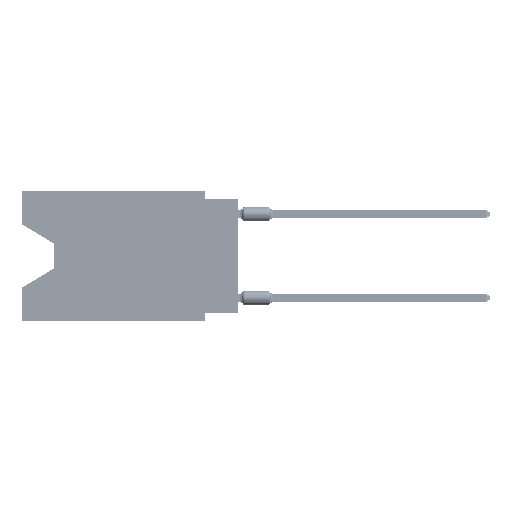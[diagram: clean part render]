
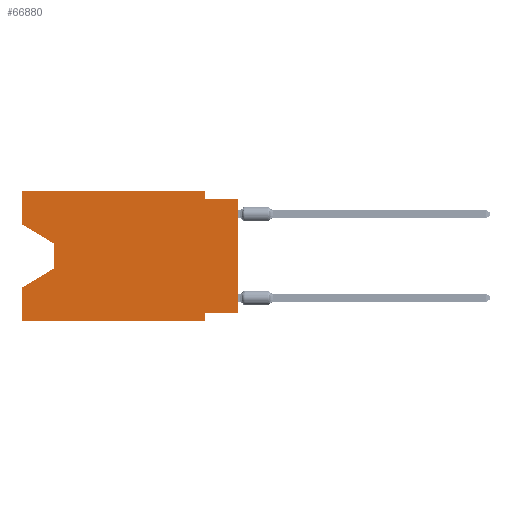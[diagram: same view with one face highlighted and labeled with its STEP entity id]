
A CAD part, left-side view. The second image highlights one B-rep face of the part: STEP entity #66880.
In plain terms, the highlighted planar face has unit normal (-1, 0, 0).
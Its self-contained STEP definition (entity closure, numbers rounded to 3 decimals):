
#413 = EDGE_CURVE ( 'NONE', #23273, #5373, #863, .T. ) ;
#863 = LINE ( 'NONE', #63190, #64928 ) ;
#1180 = DIRECTION ( 'NONE',  ( 0., 0., 1. ) ) ;
#1882 = VERTEX_POINT ( 'NONE', #2113 ) ;
#2113 = CARTESIAN_POINT ( 'NONE',  ( 0., 13.97, -5.893 ) ) ;
#4065 = EDGE_LOOP ( 'NONE', ( #66967, #74789, #69816, #65410, #41796, #32406, #82726, #46219, #72583, #57660, #9290, #78977 ) ) ;
#4071 = VECTOR ( 'NONE', #33538, 1000. ) ;
#5210 = CARTESIAN_POINT ( 'NONE',  ( 0., 16.383, -2.546 ) ) ;
#5373 = VERTEX_POINT ( 'NONE', #28654 ) ;
#8535 = VECTOR ( 'NONE', #65566, 1000. ) ;
#8777 = EDGE_CURVE ( 'NONE', #64967, #54040, #34006, .T. ) ;
#9290 = ORIENTED_EDGE ( 'NONE', *, *, #413, .F. ) ;
#9312 = VERTEX_POINT ( 'NONE', #78275 ) ;
#9584 = LINE ( 'NONE', #36928, #61810 ) ;
#10253 = VECTOR ( 'NONE', #72726, 1000. ) ;
#10540 = DIRECTION ( 'NONE',  ( 0., 0., -1. ) ) ;
#10916 = EDGE_CURVE ( 'NONE', #32950, #16256, #59727, .T. ) ;
#12124 = EDGE_CURVE ( 'NONE', #67497, #31859, #63957, .T. ) ;
#13237 = LINE ( 'NONE', #32962, #67112 ) ;
#13639 = CARTESIAN_POINT ( 'NONE',  ( 0., 0., -0.635 ) ) ;
#16256 = VERTEX_POINT ( 'NONE', #13639 ) ;
#18769 = DIRECTION ( 'NONE',  ( 0., 0., 1. ) ) ;
#19662 = DIRECTION ( 'NONE',  ( 0., -0.855, -0.519 ) ) ;
#20065 = CARTESIAN_POINT ( 'NONE',  ( 0., 16.383, 0. ) ) ;
#20564 = CARTESIAN_POINT ( 'NONE',  ( 0., 16.383, -2.546 ) ) ;
#22253 = CARTESIAN_POINT ( 'NONE',  ( 0., 2.54, -9.906 ) ) ;
#23273 = VERTEX_POINT ( 'NONE', #78458 ) ;
#23763 = FACE_OUTER_BOUND ( 'NONE', #4065, .T. ) ;
#28199 = DIRECTION ( 'NONE',  ( 0., -1., 0. ) ) ;
#28654 = CARTESIAN_POINT ( 'NONE',  ( 0., 2.54, 0. ) ) ;
#28971 = DIRECTION ( 'NONE',  ( 0., 0., -1. ) ) ;
#30026 = VECTOR ( 'NONE', #19662, 1000. ) ;
#31859 = VERTEX_POINT ( 'NONE', #34199 ) ;
#32406 = ORIENTED_EDGE ( 'NONE', *, *, #12124, .F. ) ;
#32950 = VERTEX_POINT ( 'NONE', #40521 ) ;
#32962 = CARTESIAN_POINT ( 'NONE',  ( 0., 16.383, -9.906 ) ) ;
#33538 = DIRECTION ( 'NONE',  ( 0., 0., 1. ) ) ;
#34006 = LINE ( 'NONE', #20564, #30026 ) ;
#34199 = CARTESIAN_POINT ( 'NONE',  ( 0., 2.54, -9.906 ) ) ;
#36928 = CARTESIAN_POINT ( 'NONE',  ( 0., 2.54, 0. ) ) ;
#37374 = DIRECTION ( 'NONE',  ( 0., 0., -1. ) ) ;
#38967 = CARTESIAN_POINT ( 'NONE',  ( 0., 0., -9.271 ) ) ;
#39157 = VERTEX_POINT ( 'NONE', #80428 ) ;
#40521 = CARTESIAN_POINT ( 'NONE',  ( 0., 2.54, -0.635 ) ) ;
#40680 = CARTESIAN_POINT ( 'NONE',  ( 0., 0., 0. ) ) ;
#41796 = ORIENTED_EDGE ( 'NONE', *, *, #63241, .T. ) ;
#43984 = EDGE_CURVE ( 'NONE', #39157, #67497, #69951, .T. ) ;
#44090 = EDGE_CURVE ( 'NONE', #45992, #9312, #46581, .T. ) ;
#44504 = LINE ( 'NONE', #71853, #8535 ) ;
#44846 = DIRECTION ( 'NONE',  ( 0., 0., -1. ) ) ;
#45992 = VERTEX_POINT ( 'NONE', #80542 ) ;
#46219 = ORIENTED_EDGE ( 'NONE', *, *, #68720, .T. ) ;
#46581 = LINE ( 'NONE', #52417, #74179 ) ;
#48721 = EDGE_CURVE ( 'NONE', #54040, #1882, #57646, .T. ) ;
#51124 = PLANE ( 'NONE',  #70439 ) ;
#52417 = CARTESIAN_POINT ( 'NONE',  ( 0., 16.383, 0. ) ) ;
#54040 = VERTEX_POINT ( 'NONE', #62503 ) ;
#57646 = LINE ( 'NONE', #85004, #78488 ) ;
#57660 = ORIENTED_EDGE ( 'NONE', *, *, #73236, .F. ) ;
#59727 = LINE ( 'NONE', #73168, #10253 ) ;
#59914 = VECTOR ( 'NONE', #60021, 1000. ) ;
#60021 = DIRECTION ( 'NONE',  ( 0., 1., 0. ) ) ;
#61230 = EDGE_CURVE ( 'NONE', #64967, #23273, #86924, .T. ) ;
#61810 = VECTOR ( 'NONE', #37374, 1000. ) ;
#62503 = CARTESIAN_POINT ( 'NONE',  ( 0., 13.97, -4.013 ) ) ;
#63190 = CARTESIAN_POINT ( 'NONE',  ( 0., 16.383, 0. ) ) ;
#63241 = EDGE_CURVE ( 'NONE', #45992, #31859, #13237, .T. ) ;
#63396 = CARTESIAN_POINT ( 'NONE',  ( 0., 2.54, -9.271 ) ) ;
#63957 = LINE ( 'NONE', #22253, #78878 ) ;
#64928 = VECTOR ( 'NONE', #28199, 1000. ) ;
#64967 = VERTEX_POINT ( 'NONE', #5210 ) ;
#65410 = ORIENTED_EDGE ( 'NONE', *, *, #44090, .F. ) ;
#65566 = DIRECTION ( 'NONE',  ( 0., 0.855, -0.519 ) ) ;
#66880 = ADVANCED_FACE ( 'NONE', ( #23763 ), #51124, .F. ) ;
#66967 = ORIENTED_EDGE ( 'NONE', *, *, #8777, .T. ) ;
#67112 = VECTOR ( 'NONE', #86816, 1000. ) ;
#67497 = VERTEX_POINT ( 'NONE', #63396 ) ;
#68720 = EDGE_CURVE ( 'NONE', #39157, #16256, #88652, .T. ) ;
#69816 = ORIENTED_EDGE ( 'NONE', *, *, #70245, .T. ) ;
#69951 = LINE ( 'NONE', #38967, #59914 ) ;
#70245 = EDGE_CURVE ( 'NONE', #1882, #9312, #44504, .T. ) ;
#70439 = AXIS2_PLACEMENT_3D ( 'NONE', #78469, #71735, #44846 ) ;
#71735 = DIRECTION ( 'NONE',  ( 1., 0., 0. ) ) ;
#71853 = CARTESIAN_POINT ( 'NONE',  ( 0., 13.97, -5.893 ) ) ;
#72583 = ORIENTED_EDGE ( 'NONE', *, *, #10916, .F. ) ;
#72726 = DIRECTION ( 'NONE',  ( 0., -1., 0. ) ) ;
#73168 = CARTESIAN_POINT ( 'NONE',  ( 0., 0., -0.635 ) ) ;
#73236 = EDGE_CURVE ( 'NONE', #5373, #32950, #9584, .T. ) ;
#74179 = VECTOR ( 'NONE', #18769, 1000. ) ;
#74789 = ORIENTED_EDGE ( 'NONE', *, *, #48721, .T. ) ;
#78275 = CARTESIAN_POINT ( 'NONE',  ( 0., 16.383, -7.36 ) ) ;
#78458 = CARTESIAN_POINT ( 'NONE',  ( 0., 16.383, 0. ) ) ;
#78469 = CARTESIAN_POINT ( 'NONE',  ( 0., 16.383, 0. ) ) ;
#78488 = VECTOR ( 'NONE', #10540, 1000. ) ;
#78878 = VECTOR ( 'NONE', #28971, 1000. ) ;
#78977 = ORIENTED_EDGE ( 'NONE', *, *, #61230, .F. ) ;
#79001 = VECTOR ( 'NONE', #1180, 1000. ) ;
#80428 = CARTESIAN_POINT ( 'NONE',  ( 0., 0., -9.271 ) ) ;
#80542 = CARTESIAN_POINT ( 'NONE',  ( 0., 16.383, -9.906 ) ) ;
#82726 = ORIENTED_EDGE ( 'NONE', *, *, #43984, .F. ) ;
#85004 = CARTESIAN_POINT ( 'NONE',  ( 0., 13.97, -4.013 ) ) ;
#86816 = DIRECTION ( 'NONE',  ( 0., -1., 0. ) ) ;
#86924 = LINE ( 'NONE', #20065, #4071 ) ;
#88652 = LINE ( 'NONE', #40680, #79001 ) ;
